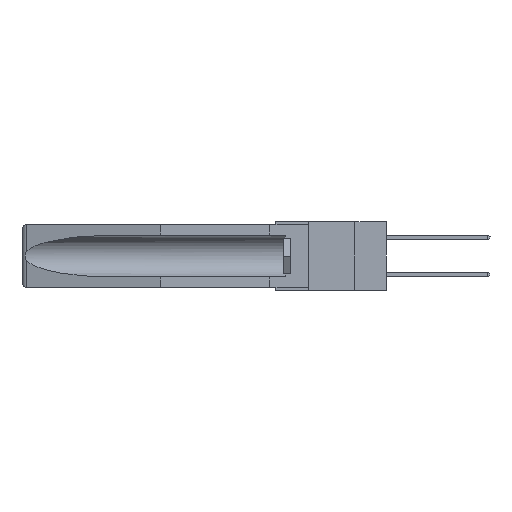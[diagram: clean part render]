
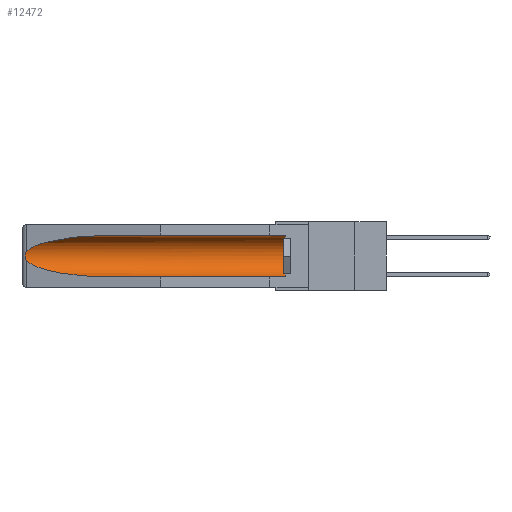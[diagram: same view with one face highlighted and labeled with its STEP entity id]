
A CAD part, left-side view. The second image highlights one B-rep face of the part: STEP entity #12472.
In plain terms, the highlighted cylindrical face has radius 2.857 mm (diameter 5.715 mm), a partial arc.
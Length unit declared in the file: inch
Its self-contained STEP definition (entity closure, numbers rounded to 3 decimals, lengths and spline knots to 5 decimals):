
#230 = EDGE_CURVE ( 'NONE', #1863, #6352, #19418, .T. ) ;
#283 = CARTESIAN_POINT ( 'NONE',  ( 0.26537, 1.52718, -0.19328 ) ) ;
#730 = CARTESIAN_POINT ( 'NONE',  ( 0.155, 1.07973, -0.284 ) ) ;
#985 = ORIENTED_EDGE ( 'NONE', *, *, #2489, .T. ) ;
#1510 = DIRECTION ( 'NONE',  ( 0., 1., 0. ) ) ;
#1863 = VERTEX_POINT ( 'NONE', #1944 ) ;
#1944 = CARTESIAN_POINT ( 'NONE',  ( 0.155, 0.126, -0.284 ) ) ;
#2489 = EDGE_CURVE ( 'NONE', #10631, #5703, #22387, .T. ) ;
#2701 = VECTOR ( 'NONE', #1510, 39.37008 ) ;
#2861 = CARTESIAN_POINT ( 'NONE',  ( 0.2673, 1.53269, -0.17917 ) ) ;
#3396 = CARTESIAN_POINT ( 'NONE',  ( 0.155, 0.126, -0.1715 ) ) ;
#5340 = CARTESIAN_POINT ( 'NONE',  ( 0.26537, 1.52718, -0.19328 ) ) ;
#5703 = VERTEX_POINT ( 'NONE', #28130 ) ;
#6352 = VERTEX_POINT ( 'NONE', #23631 ) ;
#6405 = CARTESIAN_POINT ( 'NONE',  ( 0.155, 1.07973, -0.059 ) ) ;
#6640 = CARTESIAN_POINT ( 'NONE',  ( 0.26537, 1.52718, -0.14972 ) ) ;
#7194 = EDGE_CURVE ( 'NONE', #6352, #12614, #21814, .T. ) ;
#9413 = DIRECTION ( 'NONE',  ( 0., 1., 0. ) ) ;
#9601 = CARTESIAN_POINT ( 'NONE',  ( 0.2673, 1.5327, -0.16383 ) ) ;
#10029 = CARTESIAN_POINT ( 'NONE',  ( 0.26537, 1.52718, -0.19328 ) ) ;
#10613 = CARTESIAN_POINT ( 'NONE',  ( 0.155, -0.30754, -0.284 ) ) ;
#10631 = VERTEX_POINT ( 'NONE', #5340 ) ;
#11795 = CARTESIAN_POINT ( 'NONE',  ( 0.2675, 1.53308, -0.16763 ) ) ;
#11891 = EDGE_CURVE ( 'NONE', #16206, #10631, #12812, .T. ) ;
#12472 = ADVANCED_FACE ( 'NONE', ( #20414 ), #15128, .F. ) ;
#12614 = VERTEX_POINT ( 'NONE', #6405 ) ;
#12812 = B_SPLINE_CURVE_WITH_KNOTS ( 'NONE', 3,
 ( #20612, #18534, #23043, #9601, #11795, #23243, #2861, #27615, #13902, #283 ),
 .UNSPECIFIED., .F., .F.,
 ( 4, 2, 2, 2, 4 ),
 ( 0., 0.00029, 0.00058, 0.00087, 0.00117 ),
 .UNSPECIFIED. ) ;
#13595 = DIRECTION ( 'NONE',  ( 0., 0., 1. ) ) ;
#13896 = CARTESIAN_POINT ( 'NONE',  ( 0.155, -0.30754, -0.1715 ) ) ;
#13902 = CARTESIAN_POINT ( 'NONE',  ( 0.26597, 1.5296, -0.19026 ) ) ;
#14454 = DIRECTION ( 'NONE',  ( 0., -1., 0. ) ) ;
#15128 = CYLINDRICAL_SURFACE ( 'NONE', #23929, 0.1125 ) ;
#15273 = ORIENTED_EDGE ( 'NONE', *, *, #230, .T. ) ;
#15288 = CARTESIAN_POINT ( 'NONE',  ( 0.21114, 1.30732, -0.059 ) ) ;
#15502 = CARTESIAN_POINT ( 'NONE',  ( 0.155, 1.07973, -0.059 ) ) ;
#15523 = LINE ( 'NONE', #10613, #2701 ) ;
#16206 = VERTEX_POINT ( 'NONE', #26277 ) ;
#16484 = ORIENTED_EDGE ( 'NONE', *, *, #7194, .T. ) ;
#16619 =( BOUNDED_CURVE ( )  B_SPLINE_CURVE ( 3, ( #15502, #15288, #26939, #6640 ),
 .UNSPECIFIED., .F., .F. ) 
 B_SPLINE_CURVE_WITH_KNOTS ( ( 4, 4 ),
 ( 4.71239, 6.08839 ),
 .UNSPECIFIED. ) 
 CURVE ( )  GEOMETRIC_REPRESENTATION_ITEM ( )  RATIONAL_B_SPLINE_CURVE ( ( 1., 0.848, 0.848, 1. ) ) 
 REPRESENTATION_ITEM ( '' )  );
#17280 = EDGE_CURVE ( 'NONE', #12614, #16206, #16619, .T. ) ;
#17491 = ORIENTED_EDGE ( 'NONE', *, *, #23077, .F. ) ;
#18534 = CARTESIAN_POINT ( 'NONE',  ( 0.26597, 1.52961, -0.15275 ) ) ;
#19167 = DIRECTION ( 'NONE',  ( 0., 0., 1. ) ) ;
#19418 = CIRCLE ( 'NONE', #22405, 0.1125 ) ;
#20341 = EDGE_LOOP ( 'NONE', ( #26940, #22260, #985, #17491, #15273, #16484 ) ) ;
#20414 = FACE_OUTER_BOUND ( 'NONE', #20341, .T. ) ;
#20612 = CARTESIAN_POINT ( 'NONE',  ( 0.26537, 1.52718, -0.14972 ) ) ;
#20997 = DIRECTION ( 'NONE',  ( 0., 1., 0. ) ) ;
#21814 = LINE ( 'NONE', #25435, #29266 ) ;
#22260 = ORIENTED_EDGE ( 'NONE', *, *, #11891, .T. ) ;
#22387 =( BOUNDED_CURVE ( )  B_SPLINE_CURVE ( 3, ( #10029, #27760, #25589, #730 ),
 .UNSPECIFIED., .F., .F. ) 
 B_SPLINE_CURVE_WITH_KNOTS ( ( 4, 4 ),
 ( 0.1948, 1.5708 ),
 .UNSPECIFIED. ) 
 CURVE ( )  GEOMETRIC_REPRESENTATION_ITEM ( )  RATIONAL_B_SPLINE_CURVE ( ( 1., 0.848, 0.848, 1. ) ) 
 REPRESENTATION_ITEM ( '' )  );
#22405 = AXIS2_PLACEMENT_3D ( 'NONE', #3396, #14454, #19167 ) ;
#23043 = CARTESIAN_POINT ( 'NONE',  ( 0.26654, 1.53092, -0.15636 ) ) ;
#23077 = EDGE_CURVE ( 'NONE', #1863, #5703, #15523, .T. ) ;
#23243 = CARTESIAN_POINT ( 'NONE',  ( 0.2675, 1.53308, -0.17534 ) ) ;
#23631 = CARTESIAN_POINT ( 'NONE',  ( 0.155, 0.126, -0.059 ) ) ;
#23929 = AXIS2_PLACEMENT_3D ( 'NONE', #13896, #9413, #13595 ) ;
#25435 = CARTESIAN_POINT ( 'NONE',  ( 0.155, -0.30754, -0.059 ) ) ;
#25589 = CARTESIAN_POINT ( 'NONE',  ( 0.21114, 1.30732, -0.284 ) ) ;
#26277 = CARTESIAN_POINT ( 'NONE',  ( 0.26537, 1.52718, -0.14972 ) ) ;
#26939 = CARTESIAN_POINT ( 'NONE',  ( 0.25451, 1.48313, -0.09465 ) ) ;
#26940 = ORIENTED_EDGE ( 'NONE', *, *, #17280, .T. ) ;
#27615 = CARTESIAN_POINT ( 'NONE',  ( 0.26655, 1.53094, -0.18657 ) ) ;
#27760 = CARTESIAN_POINT ( 'NONE',  ( 0.25451, 1.48313, -0.24835 ) ) ;
#28130 = CARTESIAN_POINT ( 'NONE',  ( 0.155, 1.07973, -0.284 ) ) ;
#29266 = VECTOR ( 'NONE', #20997, 39.37008 ) ;
